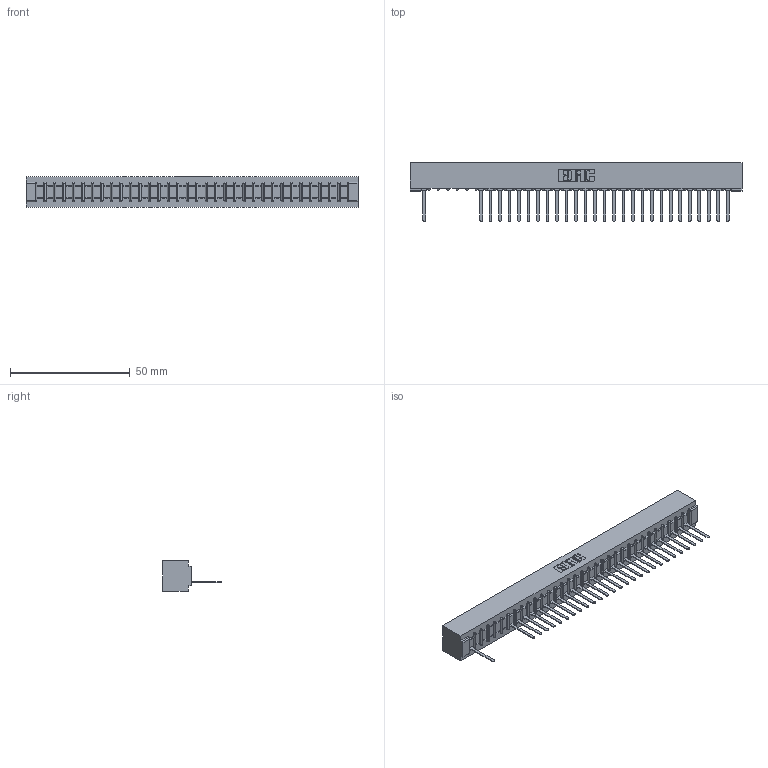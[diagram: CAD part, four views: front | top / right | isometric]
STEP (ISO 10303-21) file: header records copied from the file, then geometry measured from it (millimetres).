
FILE_DESCRIPTION (( 'STEP AP203' ), '1' );
FILE_NAME ('357-033-541-101.STEP', '2018-08-10T01:27:57', ( '' ), ( '' ), 'SwSTEP 2.0', 'SolidWorks 2016', '' );
FILE_SCHEMA (( 'CONFIG_CONTROL_DESIGN' ));
Length unit declared in the file: inch
Products named in the file (3): 307 Part_No Mounting Lugs; 307-290-002_541; 357-033-541-101
Assembly tree (29 placements, depth 2):
  357-033-541-101
    307 Part_No Mounting Lugs
    307-290-002_541  x28
Bounding box: 138.63 x 24.59 x 12.7 mm (x, y, z)
Volume: 15260.5 mm3; surface area: 18922.3 mm2
Topology: 29 solids, 29 shells, 2316 faces, 7115 edges, 4650 vertices
Faces by surface type: plane 1386, cylinder 862, sphere 68
Entity records: 29680 total; most frequent: CARTESIAN_POINT 5027, ORIENTED_EDGE 5022, DIRECTION 4881, EDGE_CURVE 2511, VECTOR 1921, LINE 1921, VERTEX_POINT 1626, AXIS2_PLACEMENT_3D 1480
